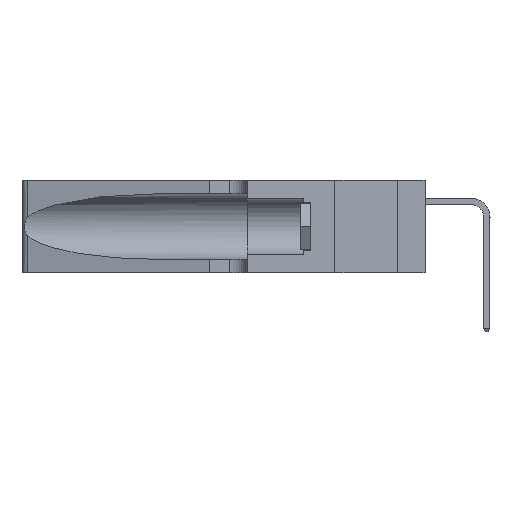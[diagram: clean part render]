
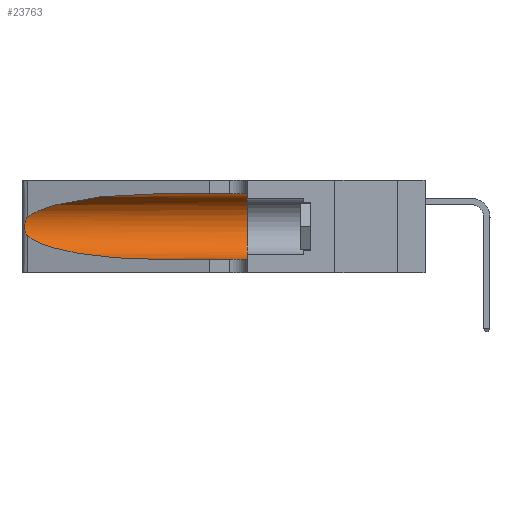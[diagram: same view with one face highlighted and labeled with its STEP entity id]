
A CAD part, left-side view. The second image highlights one B-rep face of the part: STEP entity #23763.
In plain terms, the highlighted cylindrical face has radius 3.308 mm (diameter 6.617 mm), a partial arc.
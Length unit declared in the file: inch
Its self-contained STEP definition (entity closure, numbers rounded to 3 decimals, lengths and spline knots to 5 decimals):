
#1401 = VERTEX_POINT ( 'NONE', #37420 ) ;
#1461 = VERTEX_POINT ( 'NONE', #22978 ) ;
#1612 = EDGE_CURVE ( 'NONE', #9507, #16554, #21102, .T. ) ;
#1910 = B_SPLINE_CURVE_WITH_KNOTS ( 'NONE', 3,
 ( #37878, #5290, #26150, #8393, #29135, #11383, #32105, #14352, #35053, #17331, #37998, #20317, #2554, #23305 ),
 .UNSPECIFIED., .F., .F.,
 ( 4, 2, 2, 2, 2, 2, 4 ),
 ( 0., 0.00027, 0.00053, 0.00107, 0.0016, 0.00187, 0.00214 ),
 .UNSPECIFIED. ) ;
#2284 = CARTESIAN_POINT ( 'NONE',  ( 0.18966, 0.96281, 0.31525 ) ) ;
#2554 = CARTESIAN_POINT ( 'NONE',  ( 0.25555, 1.22993, 0.14849 ) ) ;
#2766 = CARTESIAN_POINT ( 'NONE',  ( 0.1305, 0.35, 0.31525 ) ) ;
#2783 = AXIS2_PLACEMENT_3D ( 'NONE', #21146, #27092, #9344 ) ;
#3547 = VERTEX_POINT ( 'NONE', #11509 ) ;
#4432 = EDGE_LOOP ( 'NONE', ( #24811, #35008, #12811, #36888, #31359, #25819 ) ) ;
#5175 = CARTESIAN_POINT ( 'NONE',  ( 0.1305, 0.72297, 0.05475 ) ) ;
#5258 = CARTESIAN_POINT ( 'NONE',  ( 0.2373, 1.15595, 0.28018 ) ) ;
#5290 = CARTESIAN_POINT ( 'NONE',  ( 0.25555, 1.22994, 0.2215 ) ) ;
#6925 = LINE ( 'NONE', #31787, #22704 ) ;
#8393 = CARTESIAN_POINT ( 'NONE',  ( 0.25787, 1.23484, 0.2124 ) ) ;
#9344 = DIRECTION ( 'NONE',  ( 0., 0., -1. ) ) ;
#9507 = VERTEX_POINT ( 'NONE', #2766 ) ;
#10717 = EDGE_CURVE ( 'NONE', #12163, #1461, #1910, .T. ) ;
#10953 =( BOUNDED_CURVE ( )  B_SPLINE_CURVE ( 3, ( #16970, #34691, #22943, #5175 ),
 .UNSPECIFIED., .F., .F. ) 
 B_SPLINE_CURVE_WITH_KNOTS ( ( 4, 4 ),
 ( 3.44316, 4.71239 ),
 .UNSPECIFIED. ) 
 CURVE ( )  GEOMETRIC_REPRESENTATION_ITEM ( )  RATIONAL_B_SPLINE_CURVE ( ( 1., 0.87, 0.87, 1. ) ) 
 REPRESENTATION_ITEM ( '' )  );
#11383 = CARTESIAN_POINT ( 'NONE',  ( 0.26018, 1.23835, 0.19895 ) ) ;
#11509 = CARTESIAN_POINT ( 'NONE',  ( 0.1305, 0.72297, 0.31525 ) ) ;
#11920 = DIRECTION ( 'NONE',  ( 0., 1., 0. ) ) ;
#12163 = VERTEX_POINT ( 'NONE', #36238 ) ;
#12302 = AXIS2_PLACEMENT_3D ( 'NONE', #29669, #11920, #32646 ) ;
#12811 = ORIENTED_EDGE ( 'NONE', *, *, #14006, .T. ) ;
#13950 = VECTOR ( 'NONE', #34961, 39.37008 ) ;
#14006 = EDGE_CURVE ( 'NONE', #1461, #1401, #10953, .T. ) ;
#14105 = CYLINDRICAL_SURFACE ( 'NONE', #2783, 0.13025 ) ;
#14140 =( BOUNDED_CURVE ( )  B_SPLINE_CURVE ( 3, ( #20034, #2284, #5258, #25991 ),
 .UNSPECIFIED., .F., .F. ) 
 B_SPLINE_CURVE_WITH_KNOTS ( ( 4, 4 ),
 ( 1.5708, 2.84003 ),
 .UNSPECIFIED. ) 
 CURVE ( )  GEOMETRIC_REPRESENTATION_ITEM ( )  RATIONAL_B_SPLINE_CURVE ( ( 1., 0.87, 0.87, 1. ) ) 
 REPRESENTATION_ITEM ( '' )  );
#14352 = CARTESIAN_POINT ( 'NONE',  ( 0.26075, 1.23896, 0.178 ) ) ;
#14412 = CARTESIAN_POINT ( 'NONE',  ( 0.1305, 0.35, 0.05475 ) ) ;
#14634 = EDGE_CURVE ( 'NONE', #3547, #12163, #14140, .T. ) ;
#15020 = FACE_OUTER_BOUND ( 'NONE', #4432, .T. ) ;
#16554 = VERTEX_POINT ( 'NONE', #14412 ) ;
#16970 = CARTESIAN_POINT ( 'NONE',  ( 0.25487, 1.22718, 0.14631 ) ) ;
#17016 = DIRECTION ( 'NONE',  ( 0., -1., 0. ) ) ;
#17227 = CARTESIAN_POINT ( 'NONE',  ( 0.1305, 1.61858, 0.31525 ) ) ;
#17331 = CARTESIAN_POINT ( 'NONE',  ( 0.25856, 1.23593, 0.16098 ) ) ;
#20034 = CARTESIAN_POINT ( 'NONE',  ( 0.1305, 0.72297, 0.31525 ) ) ;
#20317 = CARTESIAN_POINT ( 'NONE',  ( 0.25639, 1.23186, 0.15144 ) ) ;
#21102 = CIRCLE ( 'NONE', #12302, 0.13025 ) ;
#21146 = CARTESIAN_POINT ( 'NONE',  ( 0.1305, 1.61858, 0.185 ) ) ;
#22704 = VECTOR ( 'NONE', #17016, 39.37008 ) ;
#22943 = CARTESIAN_POINT ( 'NONE',  ( 0.18966, 0.96281, 0.05475 ) ) ;
#22978 = CARTESIAN_POINT ( 'NONE',  ( 0.25487, 1.22718, 0.14631 ) ) ;
#23305 = CARTESIAN_POINT ( 'NONE',  ( 0.25487, 1.22718, 0.14631 ) ) ;
#23687 = LINE ( 'NONE', #17227, #13950 ) ;
#23763 = ADVANCED_FACE ( 'NONE', ( #15020 ), #14105, .F. ) ;
#24811 = ORIENTED_EDGE ( 'NONE', *, *, #14634, .T. ) ;
#25819 = ORIENTED_EDGE ( 'NONE', *, *, #29798, .F. ) ;
#25991 = CARTESIAN_POINT ( 'NONE',  ( 0.25487, 1.22718, 0.22369 ) ) ;
#26150 = CARTESIAN_POINT ( 'NONE',  ( 0.25639, 1.23184, 0.21858 ) ) ;
#27092 = DIRECTION ( 'NONE',  ( 0., -1., 0. ) ) ;
#29135 = CARTESIAN_POINT ( 'NONE',  ( 0.25854, 1.2359, 0.20912 ) ) ;
#29669 = CARTESIAN_POINT ( 'NONE',  ( 0.1305, 0.35, 0.185 ) ) ;
#29798 = EDGE_CURVE ( 'NONE', #3547, #9507, #23687, .T. ) ;
#30632 = EDGE_CURVE ( 'NONE', #1401, #16554, #6925, .T. ) ;
#31359 = ORIENTED_EDGE ( 'NONE', *, *, #1612, .F. ) ;
#31787 = CARTESIAN_POINT ( 'NONE',  ( 0.1305, 1.61858, 0.05475 ) ) ;
#32105 = CARTESIAN_POINT ( 'NONE',  ( 0.26075, 1.23896, 0.19203 ) ) ;
#32646 = DIRECTION ( 'NONE',  ( 0., 0., 1. ) ) ;
#34691 = CARTESIAN_POINT ( 'NONE',  ( 0.2373, 1.15595, 0.08982 ) ) ;
#34961 = DIRECTION ( 'NONE',  ( 0., -1., 0. ) ) ;
#35008 = ORIENTED_EDGE ( 'NONE', *, *, #10717, .T. ) ;
#35053 = CARTESIAN_POINT ( 'NONE',  ( 0.26017, 1.23833, 0.17102 ) ) ;
#36238 = CARTESIAN_POINT ( 'NONE',  ( 0.25487, 1.22718, 0.22369 ) ) ;
#36888 = ORIENTED_EDGE ( 'NONE', *, *, #30632, .T. ) ;
#37420 = CARTESIAN_POINT ( 'NONE',  ( 0.1305, 0.72297, 0.05475 ) ) ;
#37878 = CARTESIAN_POINT ( 'NONE',  ( 0.25487, 1.22718, 0.22369 ) ) ;
#37998 = CARTESIAN_POINT ( 'NONE',  ( 0.25789, 1.23486, 0.15765 ) ) ;
